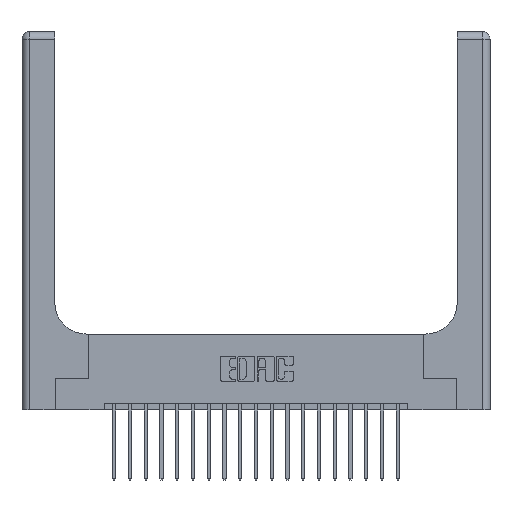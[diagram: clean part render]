
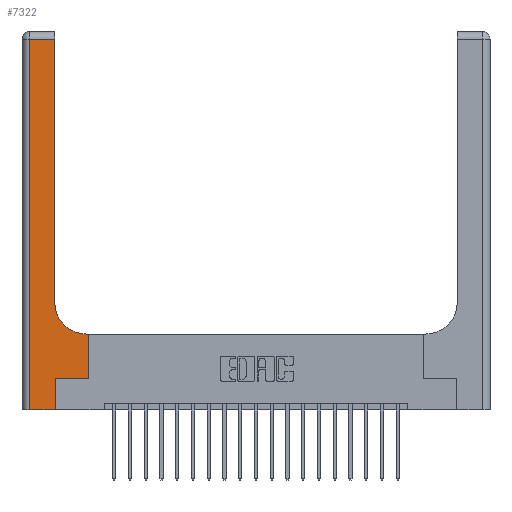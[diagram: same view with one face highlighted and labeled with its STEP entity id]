
A CAD part, top view. The second image highlights one B-rep face of the part: STEP entity #7322.
In plain terms, the highlighted planar face has unit normal (0, 0, 1).
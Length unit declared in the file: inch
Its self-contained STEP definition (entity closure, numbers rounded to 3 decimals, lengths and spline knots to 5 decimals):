
#7 = VECTOR ( 'NONE', #6493, 39.37008 ) ;
#163 = EDGE_CURVE ( 'NONE', #12218, #5547, #9875, .T. ) ;
#331 = LINE ( 'NONE', #539, #13576 ) ;
#539 = CARTESIAN_POINT ( 'NONE',  ( 0., 0., 0.37 ) ) ;
#795 = VERTEX_POINT ( 'NONE', #17358 ) ;
#1039 = CARTESIAN_POINT ( 'NONE',  ( 0.265, 0., 0.37 ) ) ;
#1439 = EDGE_CURVE ( 'NONE', #6109, #3608, #13888, .T. ) ;
#1688 = ORIENTED_EDGE ( 'NONE', *, *, #21136, .T. ) ;
#2158 = ORIENTED_EDGE ( 'NONE', *, *, #1439, .T. ) ;
#2634 = LINE ( 'NONE', #20713, #10637 ) ;
#3048 = CARTESIAN_POINT ( 'NONE',  ( 0.26, 0.85, 0.37 ) ) ;
#3219 = AXIS2_PLACEMENT_3D ( 'NONE', #8579, #9987, #15207 ) ;
#3608 = VERTEX_POINT ( 'NONE', #15755 ) ;
#3717 = LINE ( 'NONE', #19539, #4591 ) ;
#4041 = EDGE_CURVE ( 'NONE', #9343, #12218, #9415, .T. ) ;
#4102 = ORIENTED_EDGE ( 'NONE', *, *, #163, .T. ) ;
#4204 = CARTESIAN_POINT ( 'NONE',  ( 0., 2.94, 0.37 ) ) ;
#4297 = DIRECTION ( 'NONE',  ( -1., 0., 0. ) ) ;
#4364 = CARTESIAN_POINT ( 'NONE',  ( 0.06, 3., 0.37 ) ) ;
#4459 = ORIENTED_EDGE ( 'NONE', *, *, #17181, .T. ) ;
#4591 = VECTOR ( 'NONE', #19960, 39.37008 ) ;
#4902 = EDGE_CURVE ( 'NONE', #795, #7957, #2634, .T. ) ;
#5142 = DIRECTION ( 'NONE',  ( 0., 1., 0. ) ) ;
#5251 = LINE ( 'NONE', #8438, #12338 ) ;
#5506 = CARTESIAN_POINT ( 'NONE',  ( 0.26, 2.94, 0.37 ) ) ;
#5547 = VERTEX_POINT ( 'NONE', #3048 ) ;
#5694 = ORIENTED_EDGE ( 'NONE', *, *, #4902, .T. ) ;
#6109 = VERTEX_POINT ( 'NONE', #20001 ) ;
#6493 = DIRECTION ( 'NONE',  ( 0., 1., 0. ) ) ;
#6725 = DIRECTION ( 'NONE',  ( 0., 0., -1. ) ) ;
#7155 = VECTOR ( 'NONE', #4297, 39.37008 ) ;
#7304 = DIRECTION ( 'NONE',  ( 1., 0., 0. ) ) ;
#7322 = ADVANCED_FACE ( 'NONE', ( #16700 ), #13211, .F. ) ;
#7606 = CARTESIAN_POINT ( 'NONE',  ( 0.51, 0.6, 0.37 ) ) ;
#7957 = VERTEX_POINT ( 'NONE', #15498 ) ;
#8438 = CARTESIAN_POINT ( 'NONE',  ( 0.528, 0.25, 0.37 ) ) ;
#8579 = CARTESIAN_POINT ( 'NONE',  ( 0., 3., 0.37 ) ) ;
#8615 = VECTOR ( 'NONE', #20855, 39.37008 ) ;
#8976 = DIRECTION ( 'NONE',  ( 1., 0., 0. ) ) ;
#9313 = CARTESIAN_POINT ( 'NONE',  ( 0.528, 0.6, 0.37 ) ) ;
#9343 = VERTEX_POINT ( 'NONE', #9313 ) ;
#9361 = ORIENTED_EDGE ( 'NONE', *, *, #10485, .T. ) ;
#9415 = LINE ( 'NONE', #11253, #7155 ) ;
#9719 = DIRECTION ( 'NONE',  ( 1., 0., 0. ) ) ;
#9875 = CIRCLE ( 'NONE', #12645, 0.25 ) ;
#9987 = DIRECTION ( 'NONE',  ( 0., 0., -1. ) ) ;
#10485 = EDGE_CURVE ( 'NONE', #3608, #16103, #331, .T. ) ;
#10637 = VECTOR ( 'NONE', #8976, 39.37008 ) ;
#11253 = CARTESIAN_POINT ( 'NONE',  ( 0.26, 0.6, 0.37 ) ) ;
#11664 = CARTESIAN_POINT ( 'NONE',  ( 0.51, 0.85, 0.37 ) ) ;
#12218 = VERTEX_POINT ( 'NONE', #7606 ) ;
#12338 = VECTOR ( 'NONE', #5142, 39.37008 ) ;
#12645 = AXIS2_PLACEMENT_3D ( 'NONE', #11664, #6725, #9719 ) ;
#13142 = LINE ( 'NONE', #17996, #7 ) ;
#13211 = PLANE ( 'NONE',  #3219 ) ;
#13472 = EDGE_LOOP ( 'NONE', ( #1688, #15621, #2158, #9361, #4459, #5694, #14899, #13677, #4102 ) ) ;
#13576 = VECTOR ( 'NONE', #7304, 39.37008 ) ;
#13621 = VERTEX_POINT ( 'NONE', #5506 ) ;
#13677 = ORIENTED_EDGE ( 'NONE', *, *, #4041, .T. ) ;
#13888 = LINE ( 'NONE', #4364, #15384 ) ;
#14253 = LINE ( 'NONE', #4204, #8615 ) ;
#14591 = EDGE_CURVE ( 'NONE', #7957, #9343, #5251, .T. ) ;
#14899 = ORIENTED_EDGE ( 'NONE', *, *, #14591, .T. ) ;
#15207 = DIRECTION ( 'NONE',  ( -1., 0., 0. ) ) ;
#15384 = VECTOR ( 'NONE', #17281, 39.37008 ) ;
#15498 = CARTESIAN_POINT ( 'NONE',  ( 0.528, 0.25, 0.37 ) ) ;
#15621 = ORIENTED_EDGE ( 'NONE', *, *, #18931, .T. ) ;
#15755 = CARTESIAN_POINT ( 'NONE',  ( 0.06, 0., 0.37 ) ) ;
#16103 = VERTEX_POINT ( 'NONE', #1039 ) ;
#16700 = FACE_OUTER_BOUND ( 'NONE', #13472, .T. ) ;
#17181 = EDGE_CURVE ( 'NONE', #16103, #795, #13142, .T. ) ;
#17281 = DIRECTION ( 'NONE',  ( 0., -1., 0. ) ) ;
#17358 = CARTESIAN_POINT ( 'NONE',  ( 0.265, 0.25, 0.37 ) ) ;
#17996 = CARTESIAN_POINT ( 'NONE',  ( 0.265, 0., 0.37 ) ) ;
#18931 = EDGE_CURVE ( 'NONE', #13621, #6109, #14253, .T. ) ;
#19539 = CARTESIAN_POINT ( 'NONE',  ( 0.26, 3., 0.37 ) ) ;
#19960 = DIRECTION ( 'NONE',  ( 0., 1., 0. ) ) ;
#20001 = CARTESIAN_POINT ( 'NONE',  ( 0.06, 2.94, 0.37 ) ) ;
#20713 = CARTESIAN_POINT ( 'NONE',  ( 0.265, 0.25, 0.37 ) ) ;
#20855 = DIRECTION ( 'NONE',  ( -1., 0., 0. ) ) ;
#21136 = EDGE_CURVE ( 'NONE', #5547, #13621, #3717, .T. ) ;
